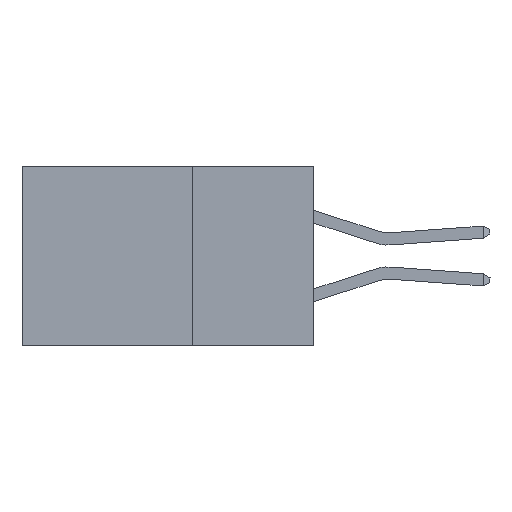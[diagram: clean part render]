
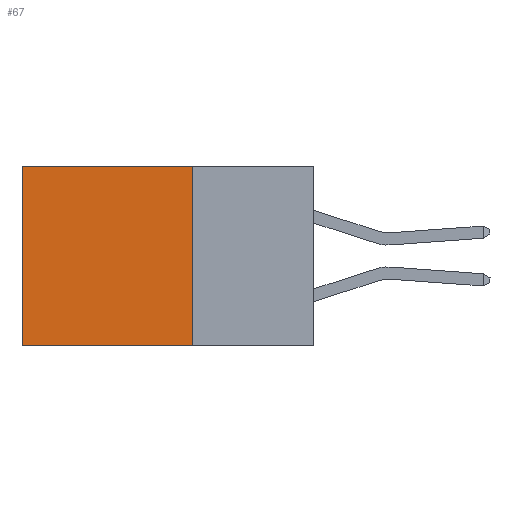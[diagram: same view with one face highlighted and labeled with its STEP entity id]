
A CAD part, left-side view. The second image highlights one B-rep face of the part: STEP entity #67.
In plain terms, the highlighted planar face has unit normal (-1, 0, 0).
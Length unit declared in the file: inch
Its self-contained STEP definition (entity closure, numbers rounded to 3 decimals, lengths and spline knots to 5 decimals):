
#67 = ADVANCED_FACE ( 'NONE', ( #23334 ), #24313, .F. ) ;
#1002 = ORIENTED_EDGE ( 'NONE', *, *, #3037, .T. ) ;
#1053 = CARTESIAN_POINT ( 'NONE',  ( 0.2875, 0.6, 0. ) ) ;
#2142 = LINE ( 'NONE', #16087, #35233 ) ;
#2789 = CARTESIAN_POINT ( 'NONE',  ( 0.2875, 0.25, -0.37 ) ) ;
#2827 = ORIENTED_EDGE ( 'NONE', *, *, #5526, .T. ) ;
#3037 = EDGE_CURVE ( 'NONE', #24866, #12341, #2142, .T. ) ;
#3409 = CARTESIAN_POINT ( 'NONE',  ( 0.2875, 0.25, 0. ) ) ;
#4267 = VERTEX_POINT ( 'NONE', #4681 ) ;
#4681 = CARTESIAN_POINT ( 'NONE',  ( 0.2875, 0.6, -0.37 ) ) ;
#4819 = VECTOR ( 'NONE', #36494, 39.37008 ) ;
#5526 = EDGE_CURVE ( 'NONE', #12341, #4267, #31800, .T. ) ;
#5812 = CARTESIAN_POINT ( 'NONE',  ( 0.2875, 0.6, 0. ) ) ;
#7382 = EDGE_CURVE ( 'NONE', #24866, #8685, #14381, .T. ) ;
#8685 = VERTEX_POINT ( 'NONE', #27227 ) ;
#12341 = VERTEX_POINT ( 'NONE', #5812 ) ;
#12381 = ORIENTED_EDGE ( 'NONE', *, *, #7382, .F. ) ;
#13443 = VECTOR ( 'NONE', #32238, 39.37008 ) ;
#14381 = LINE ( 'NONE', #39122, #29659 ) ;
#16087 = CARTESIAN_POINT ( 'NONE',  ( 0.2875, 0.25, 0. ) ) ;
#19455 = DIRECTION ( 'NONE',  ( 1., 0., 0. ) ) ;
#20364 = EDGE_LOOP ( 'NONE', ( #2827, #24698, #12381, #1002 ) ) ;
#21400 = CARTESIAN_POINT ( 'NONE',  ( 0.2875, 0.25, 0. ) ) ;
#22385 = EDGE_CURVE ( 'NONE', #8685, #4267, #37357, .T. ) ;
#22720 = DIRECTION ( 'NONE',  ( 0., 0., -1. ) ) ;
#23334 = FACE_OUTER_BOUND ( 'NONE', #20364, .T. ) ;
#24313 = PLANE ( 'NONE',  #35175 ) ;
#24698 = ORIENTED_EDGE ( 'NONE', *, *, #22385, .F. ) ;
#24866 = VERTEX_POINT ( 'NONE', #21400 ) ;
#26090 = DIRECTION ( 'NONE',  ( 0., 0., -1. ) ) ;
#27227 = CARTESIAN_POINT ( 'NONE',  ( 0.2875, 0.25, -0.37 ) ) ;
#29659 = VECTOR ( 'NONE', #26090, 39.37008 ) ;
#31800 = LINE ( 'NONE', #1053, #4819 ) ;
#32238 = DIRECTION ( 'NONE',  ( 0., 1., 0. ) ) ;
#35175 = AXIS2_PLACEMENT_3D ( 'NONE', #3409, #19455, #22720 ) ;
#35233 = VECTOR ( 'NONE', #38843, 39.37008 ) ;
#36494 = DIRECTION ( 'NONE',  ( 0., 0., -1. ) ) ;
#37357 = LINE ( 'NONE', #2789, #13443 ) ;
#38843 = DIRECTION ( 'NONE',  ( 0., 1., 0. ) ) ;
#39122 = CARTESIAN_POINT ( 'NONE',  ( 0.2875, 0.25, 0. ) ) ;
